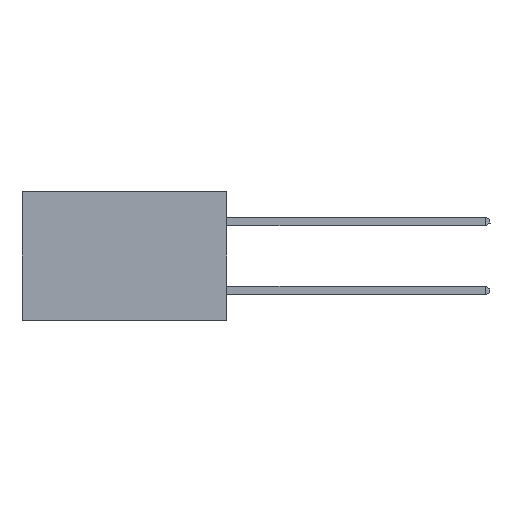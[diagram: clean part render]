
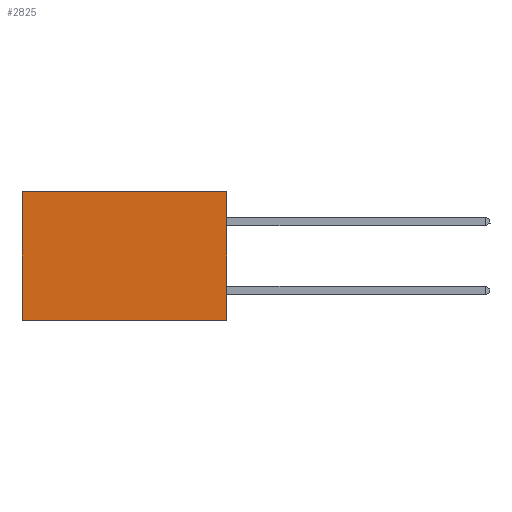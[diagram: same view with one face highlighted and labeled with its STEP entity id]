
A CAD part, left-side view. The second image highlights one B-rep face of the part: STEP entity #2825.
In plain terms, the highlighted planar face has unit normal (-1, 0, 0).
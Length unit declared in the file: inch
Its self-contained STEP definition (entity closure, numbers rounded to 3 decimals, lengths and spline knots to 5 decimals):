
#234 = LINE ( 'NONE', #2898, #4714 ) ;
#591 = ORIENTED_EDGE ( 'NONE', *, *, #5209, .F. ) ;
#704 = CARTESIAN_POINT ( 'NONE',  ( 0.277, 0.59, -0.37 ) ) ;
#935 = ORIENTED_EDGE ( 'NONE', *, *, #3988, .T. ) ;
#1230 = VERTEX_POINT ( 'NONE', #3552 ) ;
#1563 = AXIS2_PLACEMENT_3D ( 'NONE', #7599, #2896, #8351 ) ;
#2556 = EDGE_CURVE ( 'NONE', #6743, #1230, #5457, .T. ) ;
#2825 = ADVANCED_FACE ( 'NONE', ( #3008 ), #10495, .F. ) ;
#2896 = DIRECTION ( 'NONE',  ( 1., 0., 0. ) ) ;
#2898 = CARTESIAN_POINT ( 'NONE',  ( 0.277, 0., -0.37 ) ) ;
#3008 = FACE_OUTER_BOUND ( 'NONE', #5870, .T. ) ;
#3552 = CARTESIAN_POINT ( 'NONE',  ( 0.277, 0.59, -0.37 ) ) ;
#3946 = DIRECTION ( 'NONE',  ( 0., 0., -1. ) ) ;
#3988 = EDGE_CURVE ( 'NONE', #4938, #6743, #8597, .T. ) ;
#4001 = VECTOR ( 'NONE', #9468, 39.37008 ) ;
#4523 = LINE ( 'NONE', #4735, #8272 ) ;
#4524 = CARTESIAN_POINT ( 'NONE',  ( 0.277, 0.59, 0. ) ) ;
#4714 = VECTOR ( 'NONE', #6027, 39.37008 ) ;
#4735 = CARTESIAN_POINT ( 'NONE',  ( 0.277, 0., -0.37 ) ) ;
#4938 = VERTEX_POINT ( 'NONE', #6512 ) ;
#5143 = VERTEX_POINT ( 'NONE', #10439 ) ;
#5209 = EDGE_CURVE ( 'NONE', #5143, #1230, #234, .T. ) ;
#5457 = LINE ( 'NONE', #704, #9305 ) ;
#5870 = EDGE_LOOP ( 'NONE', ( #9062, #591, #9289, #935 ) ) ;
#6027 = DIRECTION ( 'NONE',  ( 0., 1., 0. ) ) ;
#6414 = CARTESIAN_POINT ( 'NONE',  ( 0.277, 0., 0. ) ) ;
#6512 = CARTESIAN_POINT ( 'NONE',  ( 0.277, 0., 0. ) ) ;
#6743 = VERTEX_POINT ( 'NONE', #4524 ) ;
#7599 = CARTESIAN_POINT ( 'NONE',  ( 0.277, 0., -0.37 ) ) ;
#8272 = VECTOR ( 'NONE', #3946, 39.37008 ) ;
#8351 = DIRECTION ( 'NONE',  ( 0., 0., -1. ) ) ;
#8597 = LINE ( 'NONE', #6414, #4001 ) ;
#9062 = ORIENTED_EDGE ( 'NONE', *, *, #2556, .T. ) ;
#9289 = ORIENTED_EDGE ( 'NONE', *, *, #9560, .F. ) ;
#9305 = VECTOR ( 'NONE', #10054, 39.37008 ) ;
#9468 = DIRECTION ( 'NONE',  ( 0., 1., 0. ) ) ;
#9560 = EDGE_CURVE ( 'NONE', #4938, #5143, #4523, .T. ) ;
#10054 = DIRECTION ( 'NONE',  ( 0., 0., -1. ) ) ;
#10439 = CARTESIAN_POINT ( 'NONE',  ( 0.277, 0., -0.37 ) ) ;
#10495 = PLANE ( 'NONE',  #1563 ) ;
